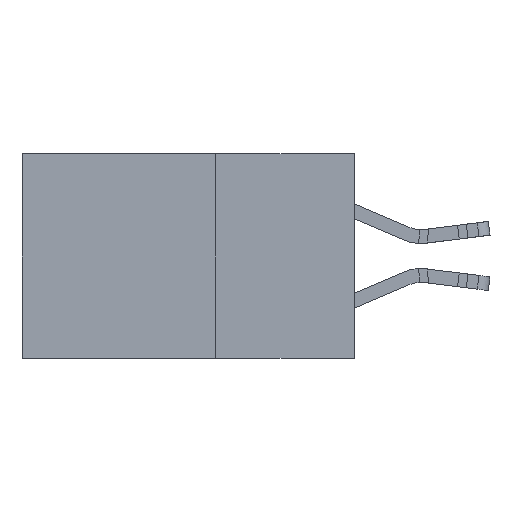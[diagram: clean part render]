
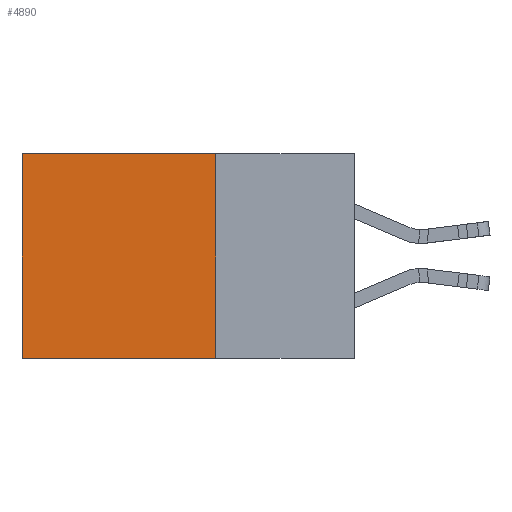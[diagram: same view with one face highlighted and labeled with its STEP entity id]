
A CAD part, left-side view. The second image highlights one B-rep face of the part: STEP entity #4890.
In plain terms, the highlighted planar face has unit normal (-1, 0, 0).
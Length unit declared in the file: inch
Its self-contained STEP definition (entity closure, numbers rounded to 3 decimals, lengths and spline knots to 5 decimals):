
#162 = DIRECTION ( 'NONE',  ( 0., 0., -1. ) ) ;
#683 = DIRECTION ( 'NONE',  ( 0., 1., 0. ) ) ;
#2080 = CARTESIAN_POINT ( 'NONE',  ( 0.2615, 0.25, -0.37 ) ) ;
#2262 = VERTEX_POINT ( 'NONE', #5520 ) ;
#3235 = CARTESIAN_POINT ( 'NONE',  ( 0.2615, 0.25, -0.37 ) ) ;
#3469 = CARTESIAN_POINT ( 'NONE',  ( 0.2615, 0.6, 0. ) ) ;
#4391 = LINE ( 'NONE', #17857, #9215 ) ;
#4890 = ADVANCED_FACE ( 'NONE', ( #12296 ), #20120, .F. ) ;
#5520 = CARTESIAN_POINT ( 'NONE',  ( 0.2615, 0.6, -0.37 ) ) ;
#5586 = CARTESIAN_POINT ( 'NONE',  ( 0.2615, 0.25, 0. ) ) ;
#6293 = EDGE_CURVE ( 'NONE', #19960, #2262, #4391, .T. ) ;
#6966 = ORIENTED_EDGE ( 'NONE', *, *, #6293, .T. ) ;
#8414 = CARTESIAN_POINT ( 'NONE',  ( 0.2615, 0.25, -0.37 ) ) ;
#9215 = VECTOR ( 'NONE', #14133, 39.37008 ) ;
#9890 = VECTOR ( 'NONE', #162, 39.37008 ) ;
#10377 = DIRECTION ( 'NONE',  ( 0., 0., -1. ) ) ;
#11928 = CARTESIAN_POINT ( 'NONE',  ( 0.2615, 0.25, -0.37 ) ) ;
#12143 = EDGE_LOOP ( 'NONE', ( #6966, #23953, #16298, #15588 ) ) ;
#12199 = VERTEX_POINT ( 'NONE', #8414 ) ;
#12296 = FACE_OUTER_BOUND ( 'NONE', #12143, .T. ) ;
#12305 = VECTOR ( 'NONE', #683, 39.37008 ) ;
#12987 = DIRECTION ( 'NONE',  ( 0., 1., 0. ) ) ;
#13651 = VECTOR ( 'NONE', #12987, 39.37008 ) ;
#13675 = AXIS2_PLACEMENT_3D ( 'NONE', #11928, #21946, #10377 ) ;
#14133 = DIRECTION ( 'NONE',  ( 0., 0., -1. ) ) ;
#15588 = ORIENTED_EDGE ( 'NONE', *, *, #17326, .T. ) ;
#16298 = ORIENTED_EDGE ( 'NONE', *, *, #18012, .F. ) ;
#17326 = EDGE_CURVE ( 'NONE', #20820, #19960, #23170, .T. ) ;
#17857 = CARTESIAN_POINT ( 'NONE',  ( 0.2615, 0.6, -0.37 ) ) ;
#18012 = EDGE_CURVE ( 'NONE', #20820, #12199, #19650, .T. ) ;
#19650 = LINE ( 'NONE', #2080, #9890 ) ;
#19960 = VERTEX_POINT ( 'NONE', #3469 ) ;
#20120 = PLANE ( 'NONE',  #13675 ) ;
#20509 = CARTESIAN_POINT ( 'NONE',  ( 0.2615, 0.25, 0. ) ) ;
#20820 = VERTEX_POINT ( 'NONE', #20509 ) ;
#21946 = DIRECTION ( 'NONE',  ( 1., 0., 0. ) ) ;
#22356 = LINE ( 'NONE', #3235, #13651 ) ;
#23170 = LINE ( 'NONE', #5586, #12305 ) ;
#23629 = EDGE_CURVE ( 'NONE', #12199, #2262, #22356, .T. ) ;
#23953 = ORIENTED_EDGE ( 'NONE', *, *, #23629, .F. ) ;
